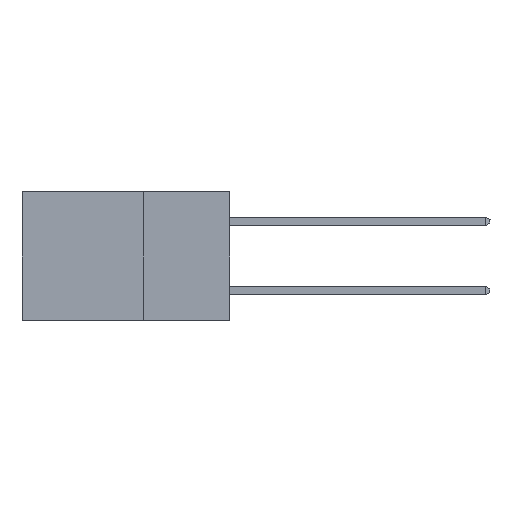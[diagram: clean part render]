
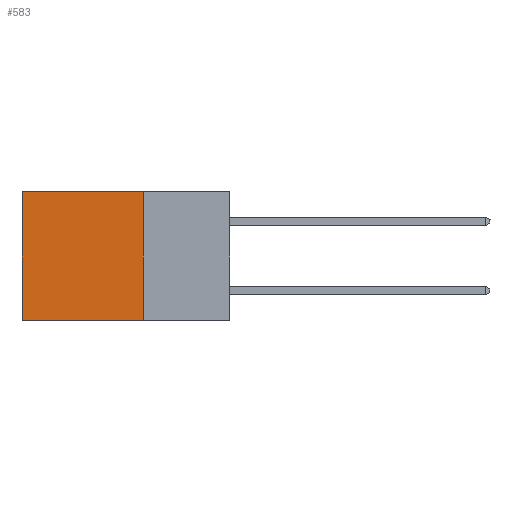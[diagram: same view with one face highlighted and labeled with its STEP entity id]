
A CAD part, left-side view. The second image highlights one B-rep face of the part: STEP entity #583.
In plain terms, the highlighted planar face has unit normal (-1, 0, 0).
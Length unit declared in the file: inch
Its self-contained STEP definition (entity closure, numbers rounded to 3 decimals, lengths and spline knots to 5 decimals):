
#150 = DIRECTION ( 'NONE',  ( 0., 0., -1. ) ) ;
#583 = ADVANCED_FACE ( 'NONE', ( #6391 ), #8100, .F. ) ;
#1405 = CARTESIAN_POINT ( 'NONE',  ( 0.2615, 0.25, -0.37 ) ) ;
#1486 = VECTOR ( 'NONE', #9662, 39.37008 ) ;
#1494 = VECTOR ( 'NONE', #2550, 39.37008 ) ;
#1913 = CARTESIAN_POINT ( 'NONE',  ( 0.2615, 0.25, -0.37 ) ) ;
#2039 = ORIENTED_EDGE ( 'NONE', *, *, #10670, .T. ) ;
#2265 = ORIENTED_EDGE ( 'NONE', *, *, #8906, .F. ) ;
#2318 = EDGE_CURVE ( 'NONE', #3740, #10087, #9969, .T. ) ;
#2550 = DIRECTION ( 'NONE',  ( 0., 0., -1. ) ) ;
#2704 = VERTEX_POINT ( 'NONE', #7538 ) ;
#3740 = VERTEX_POINT ( 'NONE', #1405 ) ;
#4435 = LINE ( 'NONE', #5262, #1494 ) ;
#4645 = EDGE_LOOP ( 'NONE', ( #2039, #5847, #2265, #5893 ) ) ;
#5153 = CARTESIAN_POINT ( 'NONE',  ( 0.2615, 0.25, 0. ) ) ;
#5185 = CARTESIAN_POINT ( 'NONE',  ( 0.2615, 0.6, -0.37 ) ) ;
#5262 = CARTESIAN_POINT ( 'NONE',  ( 0.2615, 0.25, -0.37 ) ) ;
#5847 = ORIENTED_EDGE ( 'NONE', *, *, #2318, .F. ) ;
#5893 = ORIENTED_EDGE ( 'NONE', *, *, #8351, .T. ) ;
#5949 = AXIS2_PLACEMENT_3D ( 'NONE', #9978, #8208, #150 ) ;
#6095 = LINE ( 'NONE', #5153, #1486 ) ;
#6391 = FACE_OUTER_BOUND ( 'NONE', #4645, .T. ) ;
#7538 = CARTESIAN_POINT ( 'NONE',  ( 0.2615, 0.6, 0. ) ) ;
#7931 = LINE ( 'NONE', #5185, #10912 ) ;
#8100 = PLANE ( 'NONE',  #5949 ) ;
#8208 = DIRECTION ( 'NONE',  ( 1., 0., 0. ) ) ;
#8351 = EDGE_CURVE ( 'NONE', #10354, #2704, #6095, .T. ) ;
#8906 = EDGE_CURVE ( 'NONE', #10354, #3740, #4435, .T. ) ;
#9112 = CARTESIAN_POINT ( 'NONE',  ( 0.2615, 0.25, 0. ) ) ;
#9497 = VECTOR ( 'NONE', #10963, 39.37008 ) ;
#9655 = CARTESIAN_POINT ( 'NONE',  ( 0.2615, 0.6, -0.37 ) ) ;
#9662 = DIRECTION ( 'NONE',  ( 0., 1., 0. ) ) ;
#9694 = DIRECTION ( 'NONE',  ( 0., 0., -1. ) ) ;
#9969 = LINE ( 'NONE', #1913, #9497 ) ;
#9978 = CARTESIAN_POINT ( 'NONE',  ( 0.2615, 0.25, -0.37 ) ) ;
#10087 = VERTEX_POINT ( 'NONE', #9655 ) ;
#10354 = VERTEX_POINT ( 'NONE', #9112 ) ;
#10670 = EDGE_CURVE ( 'NONE', #2704, #10087, #7931, .T. ) ;
#10912 = VECTOR ( 'NONE', #9694, 39.37008 ) ;
#10963 = DIRECTION ( 'NONE',  ( 0., 1., 0. ) ) ;
